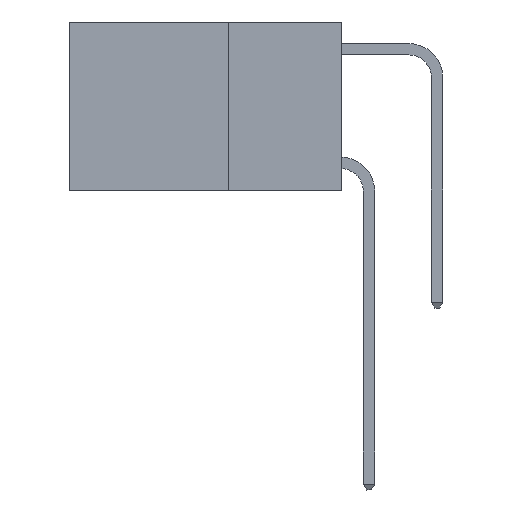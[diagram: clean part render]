
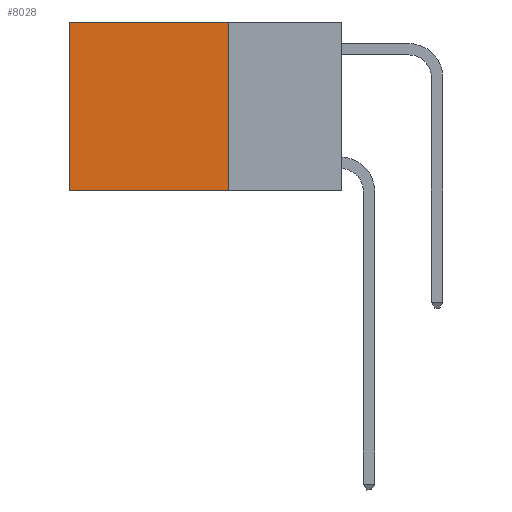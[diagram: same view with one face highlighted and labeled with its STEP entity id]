
A CAD part, left-side view. The second image highlights one B-rep face of the part: STEP entity #8028.
In plain terms, the highlighted planar face has unit normal (-1, 0, 0).
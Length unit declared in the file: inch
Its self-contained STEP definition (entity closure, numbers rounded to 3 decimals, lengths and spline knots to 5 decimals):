
#418 = DIRECTION ( 'NONE',  ( 1., 0., 0. ) ) ;
#433 = DIRECTION ( 'NONE',  ( 0., 0., -1. ) ) ;
#488 = VERTEX_POINT ( 'NONE', #10406 ) ;
#607 = CARTESIAN_POINT ( 'NONE',  ( 0.2625, 0.25, -0.37 ) ) ;
#626 = EDGE_LOOP ( 'NONE', ( #11139, #10549, #4436, #5354 ) ) ;
#646 = VECTOR ( 'NONE', #4117, 39.37008 ) ;
#1384 = LINE ( 'NONE', #9257, #646 ) ;
#1546 = VECTOR ( 'NONE', #5841, 39.37008 ) ;
#2064 = LINE ( 'NONE', #6709, #1546 ) ;
#2230 = CARTESIAN_POINT ( 'NONE',  ( 0.2625, 0.25, 0. ) ) ;
#2247 = LINE ( 'NONE', #5784, #6608 ) ;
#2332 = VECTOR ( 'NONE', #9406, 39.37008 ) ;
#2336 = AXIS2_PLACEMENT_3D ( 'NONE', #4094, #418, #11106 ) ;
#2404 = EDGE_CURVE ( 'NONE', #4303, #488, #1384, .T. ) ;
#2737 = EDGE_CURVE ( 'NONE', #8761, #488, #2247, .T. ) ;
#2944 = LINE ( 'NONE', #2230, #2332 ) ;
#3125 = PLANE ( 'NONE',  #2336 ) ;
#3143 = VERTEX_POINT ( 'NONE', #3543 ) ;
#3543 = CARTESIAN_POINT ( 'NONE',  ( 0.2625, 0.25, 0. ) ) ;
#4094 = CARTESIAN_POINT ( 'NONE',  ( 0.2625, 0.25, 0. ) ) ;
#4117 = DIRECTION ( 'NONE',  ( 0., 1., 0. ) ) ;
#4303 = VERTEX_POINT ( 'NONE', #607 ) ;
#4436 = ORIENTED_EDGE ( 'NONE', *, *, #4539, .F. ) ;
#4539 = EDGE_CURVE ( 'NONE', #3143, #4303, #2064, .T. ) ;
#5354 = ORIENTED_EDGE ( 'NONE', *, *, #6604, .T. ) ;
#5784 = CARTESIAN_POINT ( 'NONE',  ( 0.2625, 0.6, 0. ) ) ;
#5841 = DIRECTION ( 'NONE',  ( 0., 0., -1. ) ) ;
#6604 = EDGE_CURVE ( 'NONE', #3143, #8761, #2944, .T. ) ;
#6608 = VECTOR ( 'NONE', #433, 39.37008 ) ;
#6709 = CARTESIAN_POINT ( 'NONE',  ( 0.2625, 0.25, 0. ) ) ;
#7662 = CARTESIAN_POINT ( 'NONE',  ( 0.2625, 0.6, 0. ) ) ;
#8028 = ADVANCED_FACE ( 'NONE', ( #8403 ), #3125, .F. ) ;
#8403 = FACE_OUTER_BOUND ( 'NONE', #626, .T. ) ;
#8761 = VERTEX_POINT ( 'NONE', #7662 ) ;
#9257 = CARTESIAN_POINT ( 'NONE',  ( 0.2625, 0.25, -0.37 ) ) ;
#9406 = DIRECTION ( 'NONE',  ( 0., 1., 0. ) ) ;
#10406 = CARTESIAN_POINT ( 'NONE',  ( 0.2625, 0.6, -0.37 ) ) ;
#10549 = ORIENTED_EDGE ( 'NONE', *, *, #2404, .F. ) ;
#11106 = DIRECTION ( 'NONE',  ( 0., 0., -1. ) ) ;
#11139 = ORIENTED_EDGE ( 'NONE', *, *, #2737, .T. ) ;
